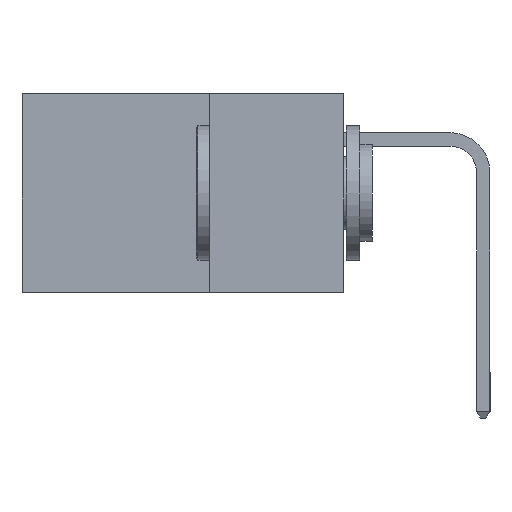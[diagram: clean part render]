
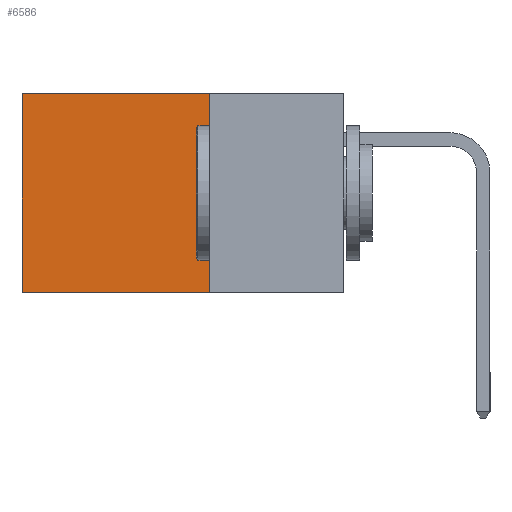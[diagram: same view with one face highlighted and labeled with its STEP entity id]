
A CAD part, left-side view. The second image highlights one B-rep face of the part: STEP entity #6586.
In plain terms, the highlighted planar face has unit normal (-1, 0, 0).
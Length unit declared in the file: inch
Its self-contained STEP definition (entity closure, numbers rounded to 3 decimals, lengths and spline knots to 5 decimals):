
#377 = EDGE_LOOP ( 'NONE', ( #10533, #9953, #11564, #675 ) ) ;
#675 = ORIENTED_EDGE ( 'NONE', *, *, #7066, .T. ) ;
#705 = CARTESIAN_POINT ( 'NONE',  ( 0.298, 0.6, 0. ) ) ;
#973 = CARTESIAN_POINT ( 'NONE',  ( 0.298, 0.6, 0. ) ) ;
#1104 = CARTESIAN_POINT ( 'NONE',  ( 0.298, 0.25, -0.37 ) ) ;
#1588 = CARTESIAN_POINT ( 'NONE',  ( 0.298, 0.25, 0. ) ) ;
#1859 = VECTOR ( 'NONE', #1951, 39.37008 ) ;
#1897 = AXIS2_PLACEMENT_3D ( 'NONE', #1588, #2404, #4353 ) ;
#1913 = CARTESIAN_POINT ( 'NONE',  ( 0.298, 0.25, 0. ) ) ;
#1932 = DIRECTION ( 'NONE',  ( 0., 0., -1. ) ) ;
#1951 = DIRECTION ( 'NONE',  ( 0., 0., -1. ) ) ;
#2404 = DIRECTION ( 'NONE',  ( 1., 0., 0. ) ) ;
#2851 = EDGE_CURVE ( 'NONE', #3930, #7007, #6532, .T. ) ;
#2905 = CARTESIAN_POINT ( 'NONE',  ( 0.298, 0.6, -0.37 ) ) ;
#2968 = VECTOR ( 'NONE', #1932, 39.37008 ) ;
#3570 = VERTEX_POINT ( 'NONE', #973 ) ;
#3930 = VERTEX_POINT ( 'NONE', #6295 ) ;
#4001 = DIRECTION ( 'NONE',  ( 0., 1., 0. ) ) ;
#4353 = DIRECTION ( 'NONE',  ( 0., 0., -1. ) ) ;
#4503 = CARTESIAN_POINT ( 'NONE',  ( 0.298, 0.25, -0.37 ) ) ;
#4513 = EDGE_CURVE ( 'NONE', #7007, #8218, #9725, .T. ) ;
#4932 = VECTOR ( 'NONE', #4001, 39.37008 ) ;
#6295 = CARTESIAN_POINT ( 'NONE',  ( 0.298, 0.25, 0. ) ) ;
#6421 = PLANE ( 'NONE',  #1897 ) ;
#6532 = LINE ( 'NONE', #1913, #1859 ) ;
#6586 = ADVANCED_FACE ( 'NONE', ( #6610 ), #6421, .F. ) ;
#6610 = FACE_OUTER_BOUND ( 'NONE', #377, .T. ) ;
#7007 = VERTEX_POINT ( 'NONE', #4503 ) ;
#7066 = EDGE_CURVE ( 'NONE', #3930, #3570, #10161, .T. ) ;
#7504 = CARTESIAN_POINT ( 'NONE',  ( 0.298, 0.25, 0. ) ) ;
#7540 = VECTOR ( 'NONE', #10606, 39.37008 ) ;
#7666 = EDGE_CURVE ( 'NONE', #3570, #8218, #8480, .T. ) ;
#8218 = VERTEX_POINT ( 'NONE', #2905 ) ;
#8480 = LINE ( 'NONE', #705, #2968 ) ;
#9725 = LINE ( 'NONE', #1104, #7540 ) ;
#9953 = ORIENTED_EDGE ( 'NONE', *, *, #4513, .F. ) ;
#10161 = LINE ( 'NONE', #7504, #4932 ) ;
#10533 = ORIENTED_EDGE ( 'NONE', *, *, #7666, .T. ) ;
#10606 = DIRECTION ( 'NONE',  ( 0., 1., 0. ) ) ;
#11564 = ORIENTED_EDGE ( 'NONE', *, *, #2851, .F. ) ;
